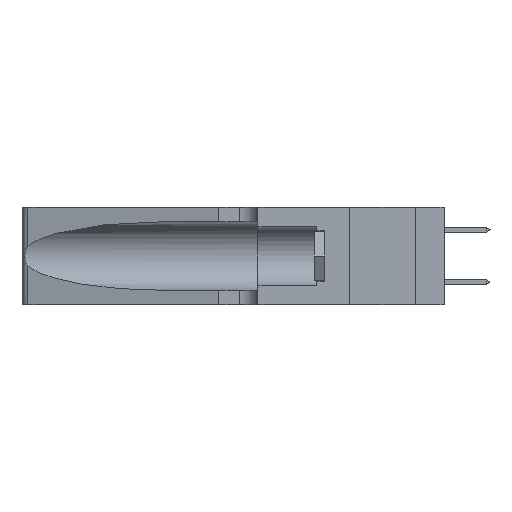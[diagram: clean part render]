
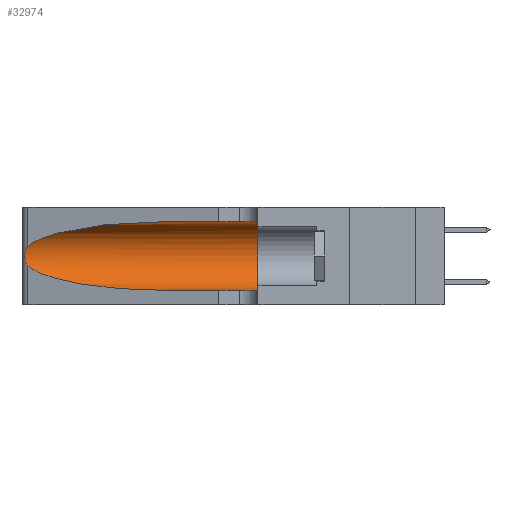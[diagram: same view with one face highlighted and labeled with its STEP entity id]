
A CAD part, left-side view. The second image highlights one B-rep face of the part: STEP entity #32974.
In plain terms, the highlighted cylindrical face has radius 3.308 mm (diameter 6.617 mm), a partial arc.
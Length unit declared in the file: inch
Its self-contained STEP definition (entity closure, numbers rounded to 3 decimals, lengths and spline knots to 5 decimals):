
#1305 =( BOUNDED_CURVE ( )  B_SPLINE_CURVE ( 3, ( #17013, #30799, #19829, #3034 ),
 .UNSPECIFIED., .F., .F. ) 
 B_SPLINE_CURVE_WITH_KNOTS ( ( 4, 4 ),
 ( 3.44316, 4.71239 ),
 .UNSPECIFIED. ) 
 CURVE ( )  GEOMETRIC_REPRESENTATION_ITEM ( )  RATIONAL_B_SPLINE_CURVE ( ( 1., 0.87, 0.87, 1. ) ) 
 REPRESENTATION_ITEM ( '' )  );
#1320 = ORIENTED_EDGE ( 'NONE', *, *, #35111, .T. ) ;
#1912 = CARTESIAN_POINT ( 'NONE',  ( 0.25487, 1.22718, 0.14631 ) ) ;
#2932 = DIRECTION ( 'NONE',  ( 0., -1., 0. ) ) ;
#3000 = CARTESIAN_POINT ( 'NONE',  ( 0.1305, 0.35, 0.05475 ) ) ;
#3034 = CARTESIAN_POINT ( 'NONE',  ( 0.1305, 0.72297, 0.05475 ) ) ;
#3299 = CARTESIAN_POINT ( 'NONE',  ( 0.1305, 1.61858, 0.05475 ) ) ;
#3545 = FACE_OUTER_BOUND ( 'NONE', #30296, .T. ) ;
#4568 = CARTESIAN_POINT ( 'NONE',  ( 0.25639, 1.23184, 0.21858 ) ) ;
#5175 = ORIENTED_EDGE ( 'NONE', *, *, #27342, .T. ) ;
#7381 = CARTESIAN_POINT ( 'NONE',  ( 0.25854, 1.2359, 0.20912 ) ) ;
#8943 = DIRECTION ( 'NONE',  ( 0., -1., 0. ) ) ;
#9652 = EDGE_CURVE ( 'NONE', #29975, #28914, #29373, .T. ) ;
#9747 = VERTEX_POINT ( 'NONE', #3000 ) ;
#10204 = CARTESIAN_POINT ( 'NONE',  ( 0.26075, 1.23896, 0.19203 ) ) ;
#10464 = CARTESIAN_POINT ( 'NONE',  ( 0.1305, 1.61858, 0.31525 ) ) ;
#12255 = ORIENTED_EDGE ( 'NONE', *, *, #9652, .F. ) ;
#13028 = CARTESIAN_POINT ( 'NONE',  ( 0.26017, 1.23833, 0.17102 ) ) ;
#13097 = VECTOR ( 'NONE', #8943, 39.37008 ) ;
#13705 = VECTOR ( 'NONE', #16730, 39.37008 ) ;
#14272 =( BOUNDED_CURVE ( )  B_SPLINE_CURVE ( 3, ( #26369, #29118, #31887, #15277 ),
 .UNSPECIFIED., .F., .F. ) 
 B_SPLINE_CURVE_WITH_KNOTS ( ( 4, 4 ),
 ( 1.5708, 2.84003 ),
 .UNSPECIFIED. ) 
 CURVE ( )  GEOMETRIC_REPRESENTATION_ITEM ( )  RATIONAL_B_SPLINE_CURVE ( ( 1., 0.87, 0.87, 1. ) ) 
 REPRESENTATION_ITEM ( '' )  );
#15277 = CARTESIAN_POINT ( 'NONE',  ( 0.25487, 1.22718, 0.22369 ) ) ;
#15714 = CARTESIAN_POINT ( 'NONE',  ( 0.25487, 1.22718, 0.22369 ) ) ;
#15837 = CARTESIAN_POINT ( 'NONE',  ( 0.25789, 1.23486, 0.15765 ) ) ;
#16027 = CARTESIAN_POINT ( 'NONE',  ( 0.1305, 0.35, 0.185 ) ) ;
#16691 = CYLINDRICAL_SURFACE ( 'NONE', #18265, 0.13025 ) ;
#16730 = DIRECTION ( 'NONE',  ( 0., -1., 0. ) ) ;
#17013 = CARTESIAN_POINT ( 'NONE',  ( 0.25487, 1.22718, 0.14631 ) ) ;
#18128 = CIRCLE ( 'NONE', #26756, 0.13025 ) ;
#18265 = AXIS2_PLACEMENT_3D ( 'NONE', #27958, #2932, #33510 ) ;
#18656 = CARTESIAN_POINT ( 'NONE',  ( 0.25555, 1.22993, 0.14849 ) ) ;
#18851 = DIRECTION ( 'NONE',  ( 0., 0., 1. ) ) ;
#19203 = CARTESIAN_POINT ( 'NONE',  ( 0.25487, 1.22718, 0.14631 ) ) ;
#19304 = VERTEX_POINT ( 'NONE', #19203 ) ;
#19829 = CARTESIAN_POINT ( 'NONE',  ( 0.18966, 0.96281, 0.05475 ) ) ;
#20335 = EDGE_CURVE ( 'NONE', #32470, #19304, #20780, .T. ) ;
#20780 = B_SPLINE_CURVE_WITH_KNOTS ( 'NONE', 3,
 ( #15714, #32335, #4568, #24113, #7381, #26914, #10204, #29645, #13028, #32451, #15837, #35235, #18656, #1912 ),
 .UNSPECIFIED., .F., .F.,
 ( 4, 2, 2, 2, 2, 2, 4 ),
 ( 0., 0.00027, 0.00053, 0.00107, 0.0016, 0.00187, 0.00214 ),
 .UNSPECIFIED. ) ;
#23195 = CARTESIAN_POINT ( 'NONE',  ( 0.1305, 0.72297, 0.31525 ) ) ;
#24113 = CARTESIAN_POINT ( 'NONE',  ( 0.25787, 1.23484, 0.2124 ) ) ;
#24352 = EDGE_CURVE ( 'NONE', #29975, #32470, #14272, .T. ) ;
#24858 = ORIENTED_EDGE ( 'NONE', *, *, #24352, .T. ) ;
#25903 = VERTEX_POINT ( 'NONE', #33266 ) ;
#26369 = CARTESIAN_POINT ( 'NONE',  ( 0.1305, 0.72297, 0.31525 ) ) ;
#26756 = AXIS2_PLACEMENT_3D ( 'NONE', #16027, #35423, #18851 ) ;
#26914 = CARTESIAN_POINT ( 'NONE',  ( 0.26018, 1.23835, 0.19895 ) ) ;
#27342 = EDGE_CURVE ( 'NONE', #19304, #25903, #1305, .T. ) ;
#27904 = LINE ( 'NONE', #3299, #13097 ) ;
#27958 = CARTESIAN_POINT ( 'NONE',  ( 0.1305, 1.61858, 0.185 ) ) ;
#28914 = VERTEX_POINT ( 'NONE', #34837 ) ;
#29065 = EDGE_CURVE ( 'NONE', #28914, #9747, #18128, .T. ) ;
#29118 = CARTESIAN_POINT ( 'NONE',  ( 0.18966, 0.96281, 0.31525 ) ) ;
#29373 = LINE ( 'NONE', #10464, #13705 ) ;
#29645 = CARTESIAN_POINT ( 'NONE',  ( 0.26075, 1.23896, 0.178 ) ) ;
#29975 = VERTEX_POINT ( 'NONE', #23195 ) ;
#30296 = EDGE_LOOP ( 'NONE', ( #24858, #33953, #5175, #1320, #31788, #12255 ) ) ;
#30799 = CARTESIAN_POINT ( 'NONE',  ( 0.2373, 1.15595, 0.08982 ) ) ;
#31212 = CARTESIAN_POINT ( 'NONE',  ( 0.25487, 1.22718, 0.22369 ) ) ;
#31788 = ORIENTED_EDGE ( 'NONE', *, *, #29065, .F. ) ;
#31887 = CARTESIAN_POINT ( 'NONE',  ( 0.2373, 1.15595, 0.28018 ) ) ;
#32335 = CARTESIAN_POINT ( 'NONE',  ( 0.25555, 1.22994, 0.2215 ) ) ;
#32451 = CARTESIAN_POINT ( 'NONE',  ( 0.25856, 1.23593, 0.16098 ) ) ;
#32470 = VERTEX_POINT ( 'NONE', #31212 ) ;
#32974 = ADVANCED_FACE ( 'NONE', ( #3545 ), #16691, .F. ) ;
#33266 = CARTESIAN_POINT ( 'NONE',  ( 0.1305, 0.72297, 0.05475 ) ) ;
#33510 = DIRECTION ( 'NONE',  ( 0., 0., -1. ) ) ;
#33953 = ORIENTED_EDGE ( 'NONE', *, *, #20335, .T. ) ;
#34837 = CARTESIAN_POINT ( 'NONE',  ( 0.1305, 0.35, 0.31525 ) ) ;
#35111 = EDGE_CURVE ( 'NONE', #25903, #9747, #27904, .T. ) ;
#35235 = CARTESIAN_POINT ( 'NONE',  ( 0.25639, 1.23186, 0.15144 ) ) ;
#35423 = DIRECTION ( 'NONE',  ( 0., 1., 0. ) ) ;
